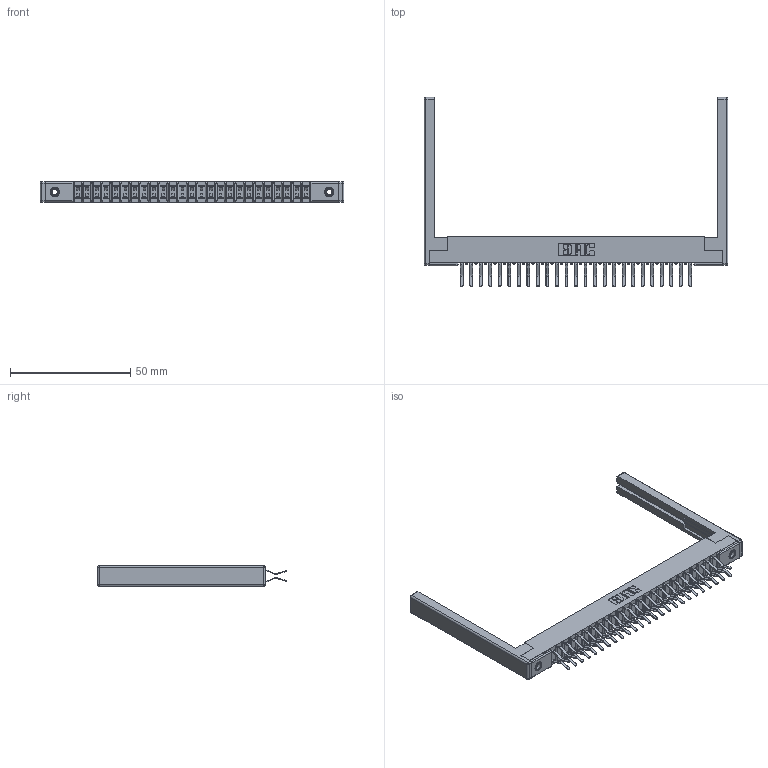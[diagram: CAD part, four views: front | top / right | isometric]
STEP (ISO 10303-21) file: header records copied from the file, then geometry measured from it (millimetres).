
FILE_DESCRIPTION (( 'STEP AP203' ), '1' );
FILE_NAME ('307-050-560-268.STEP', '2019-09-06T11:42:46', ( '' ), ( '' ), 'SwSTEP 2.0', 'SolidWorks 2016', '' );
FILE_SCHEMA (( 'CONFIG_CONTROL_DESIGN' ));
Length unit declared in the file: inch
Products named in the file (5): 345-250-001_345-250-001-102; 307-220-068; 307 Part_.156 Dia Mounting Holes; 307-050-560-268; 307-290-001_560
Assembly tree (55 placements, depth 2):
  307-050-560-268
    307 Part_.156 Dia Mounting Holes
    307-290-001_560  x50
    307-220-068  x2
    345-250-001_345-250-001-102  x2
Bounding box: 126.49 x 78.69 x 8.71 mm (x, y, z)
Volume: 12897.4 mm3; surface area: 19302.1 mm2
Topology: 55 solids, 55 shells, 2798 faces, 7813 edges, 5050 vertices
Faces by surface type: plane 1808, cylinder 914, sphere 60, cone 12, torus 4
Entity records: 27191 total; most frequent: CARTESIAN_POINT 4430, ORIENTED_EDGE 4380, DIRECTION 4362, EDGE_CURVE 2190, VECTOR 1670, LINE 1670, VERTEX_POINT 1414, AXIS2_PLACEMENT_3D 1346
